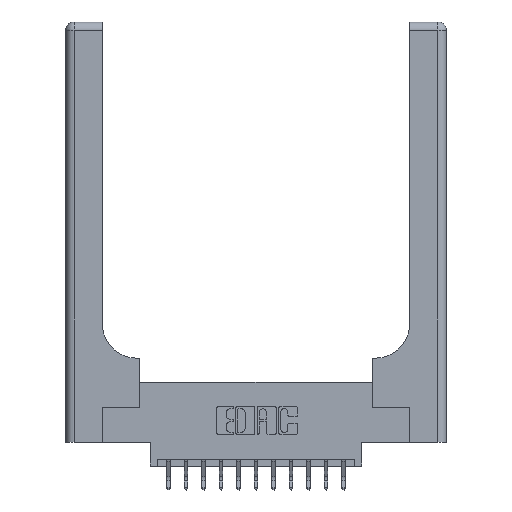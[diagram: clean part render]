
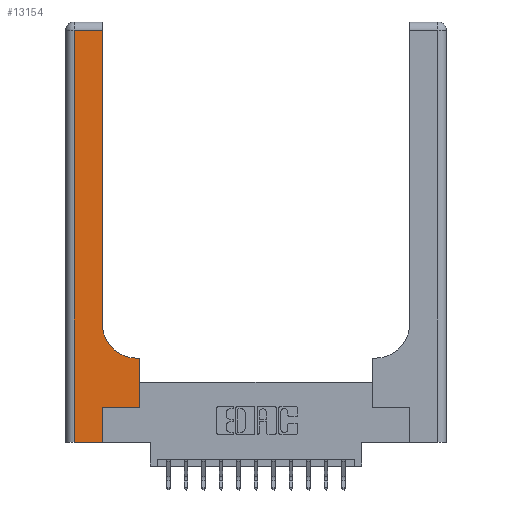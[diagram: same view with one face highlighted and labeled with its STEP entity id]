
A CAD part, top view. The second image highlights one B-rep face of the part: STEP entity #13154.
In plain terms, the highlighted planar face has unit normal (0, 0, 1).
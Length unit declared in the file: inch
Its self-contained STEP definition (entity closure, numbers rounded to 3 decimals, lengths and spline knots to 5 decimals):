
#288 = CARTESIAN_POINT ( 'NONE',  ( 0.51, 0.85, 0.37 ) ) ;
#1712 = CARTESIAN_POINT ( 'NONE',  ( 0.265, 0., 0.37 ) ) ;
#2434 = LINE ( 'NONE', #11401, #5133 ) ;
#2632 = EDGE_CURVE ( 'NONE', #13684, #7234, #11563, .T. ) ;
#2652 = CARTESIAN_POINT ( 'NONE',  ( 0.528, 0.25, 0.37 ) ) ;
#2864 = LINE ( 'NONE', #5718, #7711 ) ;
#3038 = ORIENTED_EDGE ( 'NONE', *, *, #2632, .T. ) ;
#3116 = VECTOR ( 'NONE', #8796, 39.37008 ) ;
#3486 = CIRCLE ( 'NONE', #8207, 0.25 ) ;
#3500 = VECTOR ( 'NONE', #8756, 39.37008 ) ;
#3756 = VECTOR ( 'NONE', #12882, 39.37008 ) ;
#3760 = CARTESIAN_POINT ( 'NONE',  ( 0.26, 0.85, 0.37 ) ) ;
#3868 = CARTESIAN_POINT ( 'NONE',  ( 0.26, 2.94, 0.37 ) ) ;
#4261 = ORIENTED_EDGE ( 'NONE', *, *, #14287, .T. ) ;
#4386 = VECTOR ( 'NONE', #16093, 39.37008 ) ;
#4724 = FACE_OUTER_BOUND ( 'NONE', #10645, .T. ) ;
#4816 = LINE ( 'NONE', #8817, #6306 ) ;
#4969 = PLANE ( 'NONE',  #11301 ) ;
#5006 = EDGE_CURVE ( 'NONE', #10959, #15044, #2864, .T. ) ;
#5133 = VECTOR ( 'NONE', #12879, 39.37008 ) ;
#5482 = LINE ( 'NONE', #14750, #4386 ) ;
#5718 = CARTESIAN_POINT ( 'NONE',  ( 0.528, 0.25, 0.37 ) ) ;
#5952 = LINE ( 'NONE', #14056, #3116 ) ;
#6129 = DIRECTION ( 'NONE',  ( 0., -1., 0. ) ) ;
#6306 = VECTOR ( 'NONE', #6129, 39.37008 ) ;
#6443 = LINE ( 'NONE', #14591, #8107 ) ;
#7234 = VERTEX_POINT ( 'NONE', #15434 ) ;
#7501 = CARTESIAN_POINT ( 'NONE',  ( 0., 2.94, 0.37 ) ) ;
#7711 = VECTOR ( 'NONE', #9617, 39.37008 ) ;
#7773 = CARTESIAN_POINT ( 'NONE',  ( 0.51, 0.6, 0.37 ) ) ;
#7981 = DIRECTION ( 'NONE',  ( 0., 1., 0. ) ) ;
#8107 = VECTOR ( 'NONE', #7981, 39.37008 ) ;
#8207 = AXIS2_PLACEMENT_3D ( 'NONE', #288, #10954, #14913 ) ;
#8378 = ORIENTED_EDGE ( 'NONE', *, *, #5006, .T. ) ;
#8465 = EDGE_CURVE ( 'NONE', #15222, #13684, #2434, .T. ) ;
#8756 = DIRECTION ( 'NONE',  ( 1., 0., 0. ) ) ;
#8796 = DIRECTION ( 'NONE',  ( -1., 0., 0. ) ) ;
#8817 = CARTESIAN_POINT ( 'NONE',  ( 0.06, 3., 0.37 ) ) ;
#9337 = ORIENTED_EDGE ( 'NONE', *, *, #8465, .T. ) ;
#9511 = ORIENTED_EDGE ( 'NONE', *, *, #9837, .T. ) ;
#9563 = EDGE_CURVE ( 'NONE', #15345, #12953, #6443, .T. ) ;
#9617 = DIRECTION ( 'NONE',  ( 0., 1., 0. ) ) ;
#9837 = EDGE_CURVE ( 'NONE', #15044, #11099, #5952, .T. ) ;
#10012 = DIRECTION ( 'NONE',  ( 0., 0., -1. ) ) ;
#10217 = CARTESIAN_POINT ( 'NONE',  ( 0.528, 0.6, 0.37 ) ) ;
#10258 = CARTESIAN_POINT ( 'NONE',  ( 0., 3., 0.37 ) ) ;
#10441 = VERTEX_POINT ( 'NONE', #16839 ) ;
#10645 = EDGE_LOOP ( 'NONE', ( #9337, #3038, #4261, #15769, #14257, #14446, #8378, #9511, #11036 ) ) ;
#10954 = DIRECTION ( 'NONE',  ( 0., 0., -1. ) ) ;
#10959 = VERTEX_POINT ( 'NONE', #2652 ) ;
#11036 = ORIENTED_EDGE ( 'NONE', *, *, #16784, .T. ) ;
#11099 = VERTEX_POINT ( 'NONE', #7773 ) ;
#11164 = CARTESIAN_POINT ( 'NONE',  ( 0.265, 0.25, 0.37 ) ) ;
#11301 = AXIS2_PLACEMENT_3D ( 'NONE', #10258, #10012, #17070 ) ;
#11401 = CARTESIAN_POINT ( 'NONE',  ( 0.26, 3., 0.37 ) ) ;
#11563 = LINE ( 'NONE', #7501, #3756 ) ;
#11669 = EDGE_CURVE ( 'NONE', #12953, #10959, #12982, .T. ) ;
#12879 = DIRECTION ( 'NONE',  ( 0., 1., 0. ) ) ;
#12882 = DIRECTION ( 'NONE',  ( -1., 0., 0. ) ) ;
#12884 = CARTESIAN_POINT ( 'NONE',  ( 0.265, 0.25, 0.37 ) ) ;
#12953 = VERTEX_POINT ( 'NONE', #11164 ) ;
#12982 = LINE ( 'NONE', #12884, #3500 ) ;
#13154 = ADVANCED_FACE ( 'NONE', ( #4724 ), #4969, .F. ) ;
#13684 = VERTEX_POINT ( 'NONE', #3868 ) ;
#14056 = CARTESIAN_POINT ( 'NONE',  ( 0.26, 0.6, 0.37 ) ) ;
#14257 = ORIENTED_EDGE ( 'NONE', *, *, #9563, .T. ) ;
#14287 = EDGE_CURVE ( 'NONE', #7234, #10441, #4816, .T. ) ;
#14446 = ORIENTED_EDGE ( 'NONE', *, *, #11669, .T. ) ;
#14591 = CARTESIAN_POINT ( 'NONE',  ( 0.265, 0., 0.37 ) ) ;
#14750 = CARTESIAN_POINT ( 'NONE',  ( 0., 0., 0.37 ) ) ;
#14913 = DIRECTION ( 'NONE',  ( 1., 0., 0. ) ) ;
#15044 = VERTEX_POINT ( 'NONE', #10217 ) ;
#15222 = VERTEX_POINT ( 'NONE', #3760 ) ;
#15345 = VERTEX_POINT ( 'NONE', #1712 ) ;
#15434 = CARTESIAN_POINT ( 'NONE',  ( 0.06, 2.94, 0.37 ) ) ;
#15769 = ORIENTED_EDGE ( 'NONE', *, *, #16043, .T. ) ;
#16043 = EDGE_CURVE ( 'NONE', #10441, #15345, #5482, .T. ) ;
#16093 = DIRECTION ( 'NONE',  ( 1., 0., 0. ) ) ;
#16784 = EDGE_CURVE ( 'NONE', #11099, #15222, #3486, .T. ) ;
#16839 = CARTESIAN_POINT ( 'NONE',  ( 0.06, 0., 0.37 ) ) ;
#17070 = DIRECTION ( 'NONE',  ( -1., 0., 0. ) ) ;
